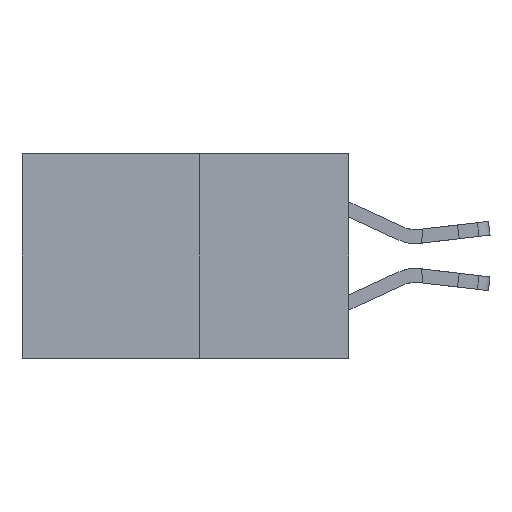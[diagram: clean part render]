
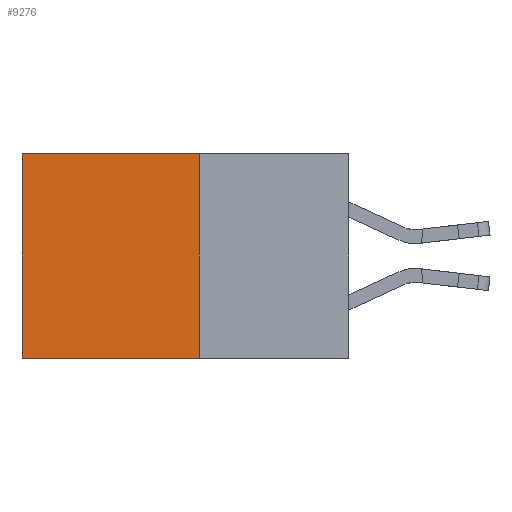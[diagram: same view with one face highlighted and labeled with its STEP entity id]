
A CAD part, left-side view. The second image highlights one B-rep face of the part: STEP entity #9276.
In plain terms, the highlighted planar face has unit normal (-1, 0, 0).
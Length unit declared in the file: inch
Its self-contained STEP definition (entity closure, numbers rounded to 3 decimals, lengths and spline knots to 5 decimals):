
#796 = VECTOR ( 'NONE', #1437, 39.37008 ) ;
#1119 = CARTESIAN_POINT ( 'NONE',  ( 0.277, 0.59, 0. ) ) ;
#1192 = CARTESIAN_POINT ( 'NONE',  ( 0.277, 0.27, -0.37 ) ) ;
#1437 = DIRECTION ( 'NONE',  ( 0., 1., 0. ) ) ;
#1617 = ORIENTED_EDGE ( 'NONE', *, *, #10982, .F. ) ;
#1664 = ORIENTED_EDGE ( 'NONE', *, *, #12707, .T. ) ;
#2300 = LINE ( 'NONE', #2403, #13788 ) ;
#2392 = CARTESIAN_POINT ( 'NONE',  ( 0.277, 0.27, 0. ) ) ;
#2403 = CARTESIAN_POINT ( 'NONE',  ( 0.277, 0.59, -0.37 ) ) ;
#2450 = DIRECTION ( 'NONE',  ( 0., 0., -1. ) ) ;
#2524 = EDGE_LOOP ( 'NONE', ( #11587, #2741, #1617, #1664 ) ) ;
#2741 = ORIENTED_EDGE ( 'NONE', *, *, #12809, .F. ) ;
#3680 = DIRECTION ( 'NONE',  ( 0., 1., 0. ) ) ;
#4408 = VERTEX_POINT ( 'NONE', #1192 ) ;
#4440 = CARTESIAN_POINT ( 'NONE',  ( 0.277, 0.27, -0.37 ) ) ;
#5019 = LINE ( 'NONE', #10398, #11271 ) ;
#5954 = VERTEX_POINT ( 'NONE', #1119 ) ;
#5989 = VERTEX_POINT ( 'NONE', #2392 ) ;
#6244 = CARTESIAN_POINT ( 'NONE',  ( 0.277, 0.27, -0.37 ) ) ;
#6689 = DIRECTION ( 'NONE',  ( 1., 0., 0. ) ) ;
#6899 = LINE ( 'NONE', #8271, #796 ) ;
#8234 = AXIS2_PLACEMENT_3D ( 'NONE', #4440, #6689, #14370 ) ;
#8271 = CARTESIAN_POINT ( 'NONE',  ( 0.277, 0.27, -0.37 ) ) ;
#8514 = VECTOR ( 'NONE', #12835, 39.37008 ) ;
#9276 = ADVANCED_FACE ( 'NONE', ( #10162 ), #11133, .F. ) ;
#9721 = CARTESIAN_POINT ( 'NONE',  ( 0.277, 0.59, -0.37 ) ) ;
#9805 = VERTEX_POINT ( 'NONE', #9721 ) ;
#10162 = FACE_OUTER_BOUND ( 'NONE', #2524, .T. ) ;
#10398 = CARTESIAN_POINT ( 'NONE',  ( 0.277, 0.27, 0. ) ) ;
#10982 = EDGE_CURVE ( 'NONE', #5989, #4408, #11808, .T. ) ;
#11133 = PLANE ( 'NONE',  #8234 ) ;
#11271 = VECTOR ( 'NONE', #3680, 39.37008 ) ;
#11587 = ORIENTED_EDGE ( 'NONE', *, *, #12686, .T. ) ;
#11808 = LINE ( 'NONE', #6244, #8514 ) ;
#12686 = EDGE_CURVE ( 'NONE', #5954, #9805, #2300, .T. ) ;
#12707 = EDGE_CURVE ( 'NONE', #5989, #5954, #5019, .T. ) ;
#12809 = EDGE_CURVE ( 'NONE', #4408, #9805, #6899, .T. ) ;
#12835 = DIRECTION ( 'NONE',  ( 0., 0., -1. ) ) ;
#13788 = VECTOR ( 'NONE', #2450, 39.37008 ) ;
#14370 = DIRECTION ( 'NONE',  ( 0., 0., -1. ) ) ;
